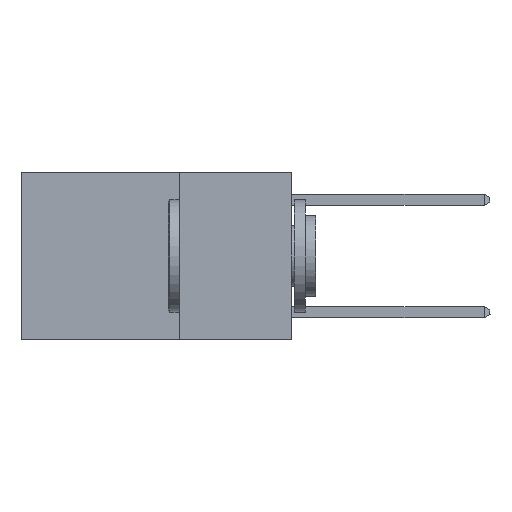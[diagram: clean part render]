
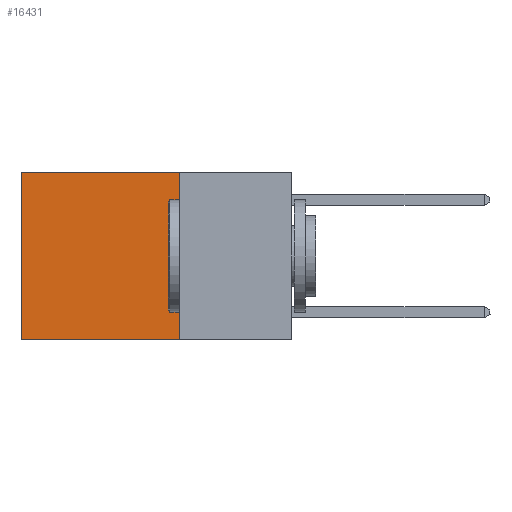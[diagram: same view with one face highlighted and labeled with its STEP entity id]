
A CAD part, left-side view. The second image highlights one B-rep face of the part: STEP entity #16431.
In plain terms, the highlighted planar face has unit normal (-1, 0, 0).
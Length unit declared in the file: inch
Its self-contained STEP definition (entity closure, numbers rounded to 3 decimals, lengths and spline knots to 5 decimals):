
#77 = EDGE_CURVE ( 'NONE', #3988, #14842, #455, .T. ) ;
#284 = VECTOR ( 'NONE', #1060, 39.37008 ) ;
#455 = LINE ( 'NONE', #3476, #9556 ) ;
#690 = DIRECTION ( 'NONE',  ( 0., 0., -1. ) ) ;
#1060 = DIRECTION ( 'NONE',  ( 0., 1., 0. ) ) ;
#1131 = FACE_OUTER_BOUND ( 'NONE', #5095, .T. ) ;
#1426 = ORIENTED_EDGE ( 'NONE', *, *, #77, .F. ) ;
#2119 = DIRECTION ( 'NONE',  ( 0., 1., 0. ) ) ;
#2806 = VERTEX_POINT ( 'NONE', #5320 ) ;
#3476 = CARTESIAN_POINT ( 'NONE',  ( 0.2625, 0.25, 0. ) ) ;
#3596 = VERTEX_POINT ( 'NONE', #15282 ) ;
#3621 = CARTESIAN_POINT ( 'NONE',  ( 0.2625, 0.6, 0. ) ) ;
#3988 = VERTEX_POINT ( 'NONE', #13275 ) ;
#4159 = EDGE_CURVE ( 'NONE', #2806, #3596, #7863, .T. ) ;
#4613 = PLANE ( 'NONE',  #6489 ) ;
#4824 = CARTESIAN_POINT ( 'NONE',  ( 0.2625, 0.25, -0.37 ) ) ;
#5095 = EDGE_LOOP ( 'NONE', ( #5226, #6348, #1426, #5360 ) ) ;
#5226 = ORIENTED_EDGE ( 'NONE', *, *, #4159, .T. ) ;
#5320 = CARTESIAN_POINT ( 'NONE',  ( 0.2625, 0.6, 0. ) ) ;
#5360 = ORIENTED_EDGE ( 'NONE', *, *, #6965, .T. ) ;
#6348 = ORIENTED_EDGE ( 'NONE', *, *, #11856, .F. ) ;
#6489 = AXIS2_PLACEMENT_3D ( 'NONE', #9130, #11698, #10368 ) ;
#6965 = EDGE_CURVE ( 'NONE', #3988, #2806, #15443, .T. ) ;
#7863 = LINE ( 'NONE', #3621, #9854 ) ;
#8237 = CARTESIAN_POINT ( 'NONE',  ( 0.2625, 0.25, 0. ) ) ;
#9130 = CARTESIAN_POINT ( 'NONE',  ( 0.2625, 0.25, 0. ) ) ;
#9232 = DIRECTION ( 'NONE',  ( 0., 0., -1. ) ) ;
#9556 = VECTOR ( 'NONE', #9232, 39.37008 ) ;
#9854 = VECTOR ( 'NONE', #690, 39.37008 ) ;
#10368 = DIRECTION ( 'NONE',  ( 0., 0., -1. ) ) ;
#11698 = DIRECTION ( 'NONE',  ( 1., 0., 0. ) ) ;
#11856 = EDGE_CURVE ( 'NONE', #14842, #3596, #12412, .T. ) ;
#12412 = LINE ( 'NONE', #16491, #16419 ) ;
#13275 = CARTESIAN_POINT ( 'NONE',  ( 0.2625, 0.25, 0. ) ) ;
#14842 = VERTEX_POINT ( 'NONE', #4824 ) ;
#15282 = CARTESIAN_POINT ( 'NONE',  ( 0.2625, 0.6, -0.37 ) ) ;
#15443 = LINE ( 'NONE', #8237, #284 ) ;
#16419 = VECTOR ( 'NONE', #2119, 39.37008 ) ;
#16431 = ADVANCED_FACE ( 'NONE', ( #1131 ), #4613, .F. ) ;
#16491 = CARTESIAN_POINT ( 'NONE',  ( 0.2625, 0.25, -0.37 ) ) ;
